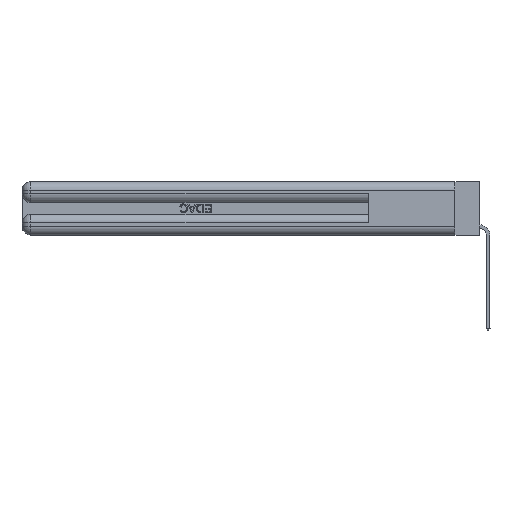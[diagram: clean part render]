
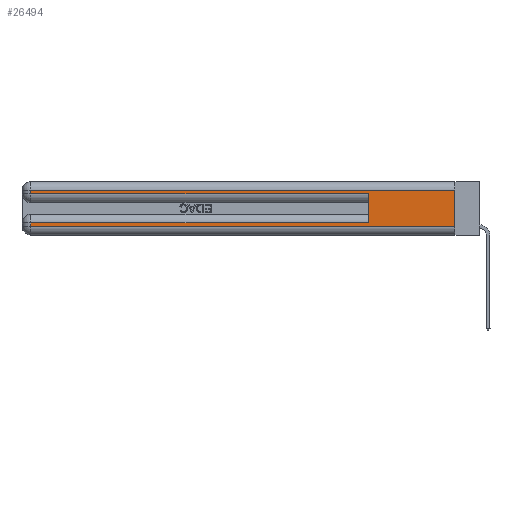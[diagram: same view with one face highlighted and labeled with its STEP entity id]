
A CAD part, left-side view. The second image highlights one B-rep face of the part: STEP entity #26494.
In plain terms, the highlighted planar face has unit normal (-1, 0, 0).
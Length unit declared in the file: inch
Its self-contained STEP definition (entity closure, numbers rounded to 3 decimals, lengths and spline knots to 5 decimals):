
#166 = CARTESIAN_POINT ( 'NONE',  ( 0., 2.94, 0.06 ) ) ;
#990 = CARTESIAN_POINT ( 'NONE',  ( 0., 0., 0.06 ) ) ;
#1203 = VERTEX_POINT ( 'NONE', #7337 ) ;
#1422 = FACE_OUTER_BOUND ( 'NONE', #25915, .T. ) ;
#1519 = EDGE_CURVE ( 'NONE', #9243, #12631, #7280, .T. ) ;
#1802 = DIRECTION ( 'NONE',  ( 0., 1., 0. ) ) ;
#2234 = EDGE_CURVE ( 'NONE', #11034, #25241, #12579, .T. ) ;
#2302 = CARTESIAN_POINT ( 'NONE',  ( 0., 0.6, 0.285 ) ) ;
#3032 = CARTESIAN_POINT ( 'NONE',  ( 0., 0., 0.06 ) ) ;
#3088 = EDGE_CURVE ( 'NONE', #21459, #13173, #24370, .T. ) ;
#3461 = CARTESIAN_POINT ( 'NONE',  ( 0., 0., 0.31 ) ) ;
#4868 = ORIENTED_EDGE ( 'NONE', *, *, #19507, .T. ) ;
#4880 = DIRECTION ( 'NONE',  ( 0., -1., 0. ) ) ;
#5376 = VECTOR ( 'NONE', #7215, 39.37008 ) ;
#6343 = CARTESIAN_POINT ( 'NONE',  ( 0., 0., 0.085 ) ) ;
#7104 = VECTOR ( 'NONE', #26183, 39.37008 ) ;
#7142 = LINE ( 'NONE', #21422, #24506 ) ;
#7215 = DIRECTION ( 'NONE',  ( 0., 0., -1. ) ) ;
#7280 = LINE ( 'NONE', #990, #21056 ) ;
#7337 = CARTESIAN_POINT ( 'NONE',  ( 0., 0., 0.31 ) ) ;
#7461 = CARTESIAN_POINT ( 'NONE',  ( 0., 0., 0.285 ) ) ;
#8118 = LINE ( 'NONE', #3461, #16139 ) ;
#8458 = CARTESIAN_POINT ( 'NONE',  ( 0., 2.94, 0.37 ) ) ;
#8718 = LINE ( 'NONE', #8458, #5376 ) ;
#9179 = LINE ( 'NONE', #21686, #15768 ) ;
#9243 = VERTEX_POINT ( 'NONE', #166 ) ;
#9589 = DIRECTION ( 'NONE',  ( 1., 0., 0. ) ) ;
#9855 = PLANE ( 'NONE',  #22612 ) ;
#9993 = ORIENTED_EDGE ( 'NONE', *, *, #3088, .T. ) ;
#11034 = VERTEX_POINT ( 'NONE', #19057 ) ;
#11180 = DIRECTION ( 'NONE',  ( 0., 0., 1. ) ) ;
#11623 = DIRECTION ( 'NONE',  ( 0., 1., 0. ) ) ;
#12004 = EDGE_CURVE ( 'NONE', #1203, #12631, #9179, .T. ) ;
#12025 = VECTOR ( 'NONE', #22700, 39.37008 ) ;
#12061 = VECTOR ( 'NONE', #1802, 39.37008 ) ;
#12579 = LINE ( 'NONE', #20277, #12025 ) ;
#12631 = VERTEX_POINT ( 'NONE', #3032 ) ;
#13104 = EDGE_CURVE ( 'NONE', #21459, #18745, #7142, .T. ) ;
#13173 = VERTEX_POINT ( 'NONE', #15726 ) ;
#13464 = CARTESIAN_POINT ( 'NONE',  ( 0., 0.6, 0.085 ) ) ;
#13962 = CARTESIAN_POINT ( 'NONE',  ( 0., 2.94, 0.285 ) ) ;
#14208 = ORIENTED_EDGE ( 'NONE', *, *, #19930, .T. ) ;
#14834 = ORIENTED_EDGE ( 'NONE', *, *, #2234, .T. ) ;
#15726 = CARTESIAN_POINT ( 'NONE',  ( 0., 2.94, 0.085 ) ) ;
#15768 = VECTOR ( 'NONE', #17636, 39.37008 ) ;
#16139 = VECTOR ( 'NONE', #11623, 39.37008 ) ;
#16734 = EDGE_CURVE ( 'NONE', #13173, #9243, #8718, .T. ) ;
#17636 = DIRECTION ( 'NONE',  ( 0., 0., -1. ) ) ;
#18745 = VERTEX_POINT ( 'NONE', #2302 ) ;
#19057 = CARTESIAN_POINT ( 'NONE',  ( 0., 2.94, 0.31 ) ) ;
#19507 = EDGE_CURVE ( 'NONE', #25241, #18745, #22011, .T. ) ;
#19930 = EDGE_CURVE ( 'NONE', #1203, #11034, #8118, .T. ) ;
#19944 = CARTESIAN_POINT ( 'NONE',  ( 0., 0., 0.37 ) ) ;
#20277 = CARTESIAN_POINT ( 'NONE',  ( 0., 2.94, 0.37 ) ) ;
#21056 = VECTOR ( 'NONE', #4880, 39.37008 ) ;
#21154 = ORIENTED_EDGE ( 'NONE', *, *, #12004, .F. ) ;
#21325 = ORIENTED_EDGE ( 'NONE', *, *, #13104, .F. ) ;
#21422 = CARTESIAN_POINT ( 'NONE',  ( 0., 0.6, 0.145 ) ) ;
#21459 = VERTEX_POINT ( 'NONE', #13464 ) ;
#21686 = CARTESIAN_POINT ( 'NONE',  ( 0., 0., 0.37 ) ) ;
#22011 = LINE ( 'NONE', #7461, #7104 ) ;
#22612 = AXIS2_PLACEMENT_3D ( 'NONE', #19944, #9589, #26541 ) ;
#22700 = DIRECTION ( 'NONE',  ( 0., 0., -1. ) ) ;
#23198 = ORIENTED_EDGE ( 'NONE', *, *, #16734, .T. ) ;
#24370 = LINE ( 'NONE', #6343, #12061 ) ;
#24506 = VECTOR ( 'NONE', #11180, 39.37008 ) ;
#25241 = VERTEX_POINT ( 'NONE', #13962 ) ;
#25915 = EDGE_LOOP ( 'NONE', ( #21154, #14208, #14834, #4868, #21325, #9993, #23198, #25944 ) ) ;
#25944 = ORIENTED_EDGE ( 'NONE', *, *, #1519, .T. ) ;
#26183 = DIRECTION ( 'NONE',  ( 0., -1., 0. ) ) ;
#26494 = ADVANCED_FACE ( 'NONE', ( #1422 ), #9855, .F. ) ;
#26541 = DIRECTION ( 'NONE',  ( 0., 0., -1. ) ) ;
